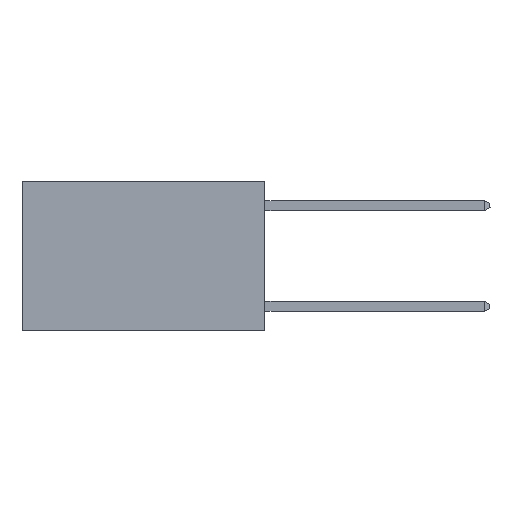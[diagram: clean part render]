
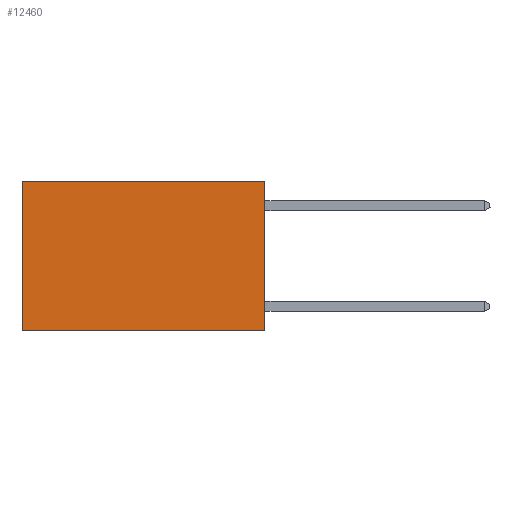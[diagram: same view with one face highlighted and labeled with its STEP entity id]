
A CAD part, left-side view. The second image highlights one B-rep face of the part: STEP entity #12460.
In plain terms, the highlighted planar face has unit normal (-1, 0, 0).
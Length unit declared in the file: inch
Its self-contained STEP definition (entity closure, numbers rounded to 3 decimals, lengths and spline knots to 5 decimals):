
#346 = VERTEX_POINT ( 'NONE', #17605 ) ;
#614 = CARTESIAN_POINT ( 'NONE',  ( 0.2625, 0.6, 0. ) ) ;
#1059 = EDGE_CURVE ( 'NONE', #346, #17540, #7826, .T. ) ;
#1180 = CARTESIAN_POINT ( 'NONE',  ( 0.2625, 0.6, 0. ) ) ;
#1714 = ORIENTED_EDGE ( 'NONE', *, *, #16366, .T. ) ;
#2711 = CARTESIAN_POINT ( 'NONE',  ( 0.2625, 0., 0. ) ) ;
#2969 = VERTEX_POINT ( 'NONE', #1180 ) ;
#4119 = CARTESIAN_POINT ( 'NONE',  ( 0.2625, 0., 0. ) ) ;
#4855 = DIRECTION ( 'NONE',  ( 0., 1., 0. ) ) ;
#5393 = DIRECTION ( 'NONE',  ( 1., 0., 0. ) ) ;
#5440 = VERTEX_POINT ( 'NONE', #18363 ) ;
#5544 = EDGE_CURVE ( 'NONE', #5440, #346, #17048, .T. ) ;
#6294 = FACE_OUTER_BOUND ( 'NONE', #11046, .T. ) ;
#6408 = CARTESIAN_POINT ( 'NONE',  ( 0.2625, 0., -0.37 ) ) ;
#7548 = CARTESIAN_POINT ( 'NONE',  ( 0.2625, 0., 0. ) ) ;
#7822 = DIRECTION ( 'NONE',  ( 0., 0., -1. ) ) ;
#7826 = LINE ( 'NONE', #6408, #13310 ) ;
#8058 = VECTOR ( 'NONE', #4855, 39.37008 ) ;
#8293 = VECTOR ( 'NONE', #7822, 39.37008 ) ;
#9018 = VECTOR ( 'NONE', #11371, 39.37008 ) ;
#10783 = DIRECTION ( 'NONE',  ( 0., 1., 0. ) ) ;
#10807 = ORIENTED_EDGE ( 'NONE', *, *, #14369, .T. ) ;
#11046 = EDGE_LOOP ( 'NONE', ( #1714, #12280, #16771, #10807 ) ) ;
#11371 = DIRECTION ( 'NONE',  ( 0., 0., -1. ) ) ;
#12280 = ORIENTED_EDGE ( 'NONE', *, *, #1059, .F. ) ;
#12460 = ADVANCED_FACE ( 'NONE', ( #6294 ), #18756, .F. ) ;
#13310 = VECTOR ( 'NONE', #10783, 39.37008 ) ;
#14238 = LINE ( 'NONE', #614, #8293 ) ;
#14315 = DIRECTION ( 'NONE',  ( 0., 0., -1. ) ) ;
#14369 = EDGE_CURVE ( 'NONE', #5440, #2969, #18125, .T. ) ;
#15318 = CARTESIAN_POINT ( 'NONE',  ( 0.2625, 0.6, -0.37 ) ) ;
#16366 = EDGE_CURVE ( 'NONE', #2969, #17540, #14238, .T. ) ;
#16771 = ORIENTED_EDGE ( 'NONE', *, *, #5544, .F. ) ;
#17048 = LINE ( 'NONE', #2711, #9018 ) ;
#17540 = VERTEX_POINT ( 'NONE', #15318 ) ;
#17571 = AXIS2_PLACEMENT_3D ( 'NONE', #4119, #5393, #14315 ) ;
#17605 = CARTESIAN_POINT ( 'NONE',  ( 0.2625, 0., -0.37 ) ) ;
#18125 = LINE ( 'NONE', #7548, #8058 ) ;
#18363 = CARTESIAN_POINT ( 'NONE',  ( 0.2625, 0., 0. ) ) ;
#18756 = PLANE ( 'NONE',  #17571 ) ;
